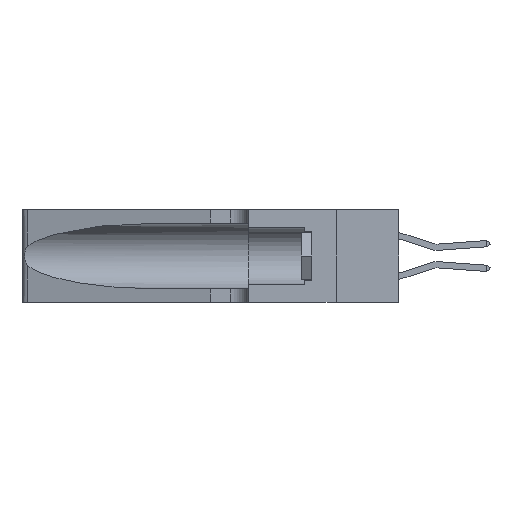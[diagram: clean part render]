
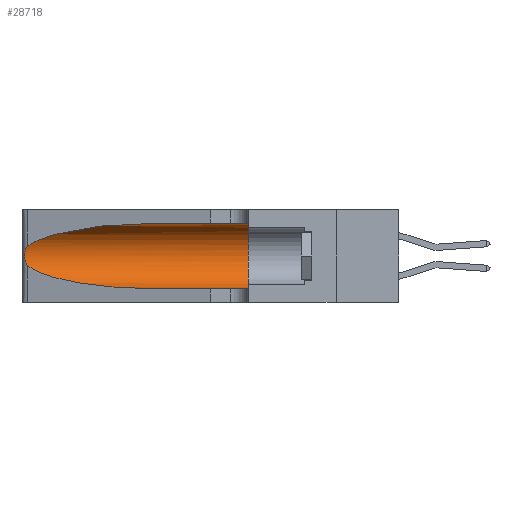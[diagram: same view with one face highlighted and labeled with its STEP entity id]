
A CAD part, left-side view. The second image highlights one B-rep face of the part: STEP entity #28718.
In plain terms, the highlighted cylindrical face has radius 3.308 mm (diameter 6.617 mm), a partial arc.
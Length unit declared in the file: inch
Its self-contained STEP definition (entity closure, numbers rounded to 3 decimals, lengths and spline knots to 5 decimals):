
#351 = VERTEX_POINT ( 'NONE', #17023 ) ;
#1163 = EDGE_CURVE ( 'NONE', #14484, #18772, #7577, .T. ) ;
#1216 = ORIENTED_EDGE ( 'NONE', *, *, #2933, .T. ) ;
#1233 = CARTESIAN_POINT ( 'NONE',  ( 0.1305, 1.61858, 0.05475 ) ) ;
#2181 = CARTESIAN_POINT ( 'NONE',  ( 0.25854, 1.2359, 0.20912 ) ) ;
#2210 = EDGE_LOOP ( 'NONE', ( #8431, #28573, #1216, #13275, #25528, #15955 ) ) ;
#2351 = DIRECTION ( 'NONE',  ( 0., -1., 0. ) ) ;
#2374 = CARTESIAN_POINT ( 'NONE',  ( 0.25487, 1.22718, 0.14631 ) ) ;
#2444 = EDGE_CURVE ( 'NONE', #351, #23136, #7590, .T. ) ;
#2933 = EDGE_CURVE ( 'NONE', #22649, #6682, #25828, .T. ) ;
#4536 = CARTESIAN_POINT ( 'NONE',  ( 0.26075, 1.23896, 0.19203 ) ) ;
#4545 = CARTESIAN_POINT ( 'NONE',  ( 0.2373, 1.15595, 0.28018 ) ) ;
#5528 = CARTESIAN_POINT ( 'NONE',  ( 0.1305, 0.72297, 0.31525 ) ) ;
#6630 = EDGE_CURVE ( 'NONE', #14484, #351, #11268, .T. ) ;
#6682 = VERTEX_POINT ( 'NONE', #26840 ) ;
#6856 = CARTESIAN_POINT ( 'NONE',  ( 0.26017, 1.23833, 0.17102 ) ) ;
#7577 =( BOUNDED_CURVE ( )  B_SPLINE_CURVE ( 3, ( #5528, #20667, #4545, #17344 ),
 .UNSPECIFIED., .F., .F. ) 
 B_SPLINE_CURVE_WITH_KNOTS ( ( 4, 4 ),
 ( 1.5708, 2.84003 ),
 .UNSPECIFIED. ) 
 CURVE ( )  GEOMETRIC_REPRESENTATION_ITEM ( )  RATIONAL_B_SPLINE_CURVE ( ( 1., 0.87, 0.87, 1. ) ) 
 REPRESENTATION_ITEM ( '' )  );
#7590 = CIRCLE ( 'NONE', #27011, 0.13025 ) ;
#8431 = ORIENTED_EDGE ( 'NONE', *, *, #1163, .T. ) ;
#9037 = CARTESIAN_POINT ( 'NONE',  ( 0.25555, 1.22994, 0.2215 ) ) ;
#9132 = CARTESIAN_POINT ( 'NONE',  ( 0.25789, 1.23486, 0.15765 ) ) ;
#10758 = LINE ( 'NONE', #1233, #16496 ) ;
#11268 = LINE ( 'NONE', #13593, #21477 ) ;
#11364 = CARTESIAN_POINT ( 'NONE',  ( 0.25555, 1.22993, 0.14849 ) ) ;
#11855 = AXIS2_PLACEMENT_3D ( 'NONE', #19155, #14835, #17044 ) ;
#13043 = DIRECTION ( 'NONE',  ( 0., 0., 1. ) ) ;
#13275 = ORIENTED_EDGE ( 'NONE', *, *, #23592, .T. ) ;
#13399 = CARTESIAN_POINT ( 'NONE',  ( 0.1305, 0.35, 0.185 ) ) ;
#13593 = CARTESIAN_POINT ( 'NONE',  ( 0.1305, 1.61858, 0.31525 ) ) ;
#13814 = CARTESIAN_POINT ( 'NONE',  ( 0.25487, 1.22718, 0.22369 ) ) ;
#14484 = VERTEX_POINT ( 'NONE', #27884 ) ;
#14698 = DIRECTION ( 'NONE',  ( 0., -1., 0. ) ) ;
#14835 = DIRECTION ( 'NONE',  ( 0., -1., 0. ) ) ;
#15591 = CARTESIAN_POINT ( 'NONE',  ( 0.25787, 1.23484, 0.2124 ) ) ;
#15955 = ORIENTED_EDGE ( 'NONE', *, *, #6630, .F. ) ;
#16496 = VECTOR ( 'NONE', #14698, 39.37008 ) ;
#17023 = CARTESIAN_POINT ( 'NONE',  ( 0.1305, 0.35, 0.31525 ) ) ;
#17044 = DIRECTION ( 'NONE',  ( 0., 0., -1. ) ) ;
#17193 = EDGE_CURVE ( 'NONE', #18772, #22649, #18629, .T. ) ;
#17344 = CARTESIAN_POINT ( 'NONE',  ( 0.25487, 1.22718, 0.22369 ) ) ;
#17785 = CARTESIAN_POINT ( 'NONE',  ( 0.26018, 1.23835, 0.19895 ) ) ;
#18629 = B_SPLINE_CURVE_WITH_KNOTS ( 'NONE', 3,
 ( #24306, #9037, #28663, #15591, #2181, #17785, #4536, #19994, #6856, #22212, #9132, #24398, #11364, #26594 ),
 .UNSPECIFIED., .F., .F.,
 ( 4, 2, 2, 2, 2, 2, 4 ),
 ( 0., 0.00027, 0.00053, 0.00107, 0.0016, 0.00187, 0.00214 ),
 .UNSPECIFIED. ) ;
#18772 = VERTEX_POINT ( 'NONE', #13814 ) ;
#19155 = CARTESIAN_POINT ( 'NONE',  ( 0.1305, 1.61858, 0.185 ) ) ;
#19795 = CARTESIAN_POINT ( 'NONE',  ( 0.1305, 0.35, 0.05475 ) ) ;
#19994 = CARTESIAN_POINT ( 'NONE',  ( 0.26075, 1.23896, 0.178 ) ) ;
#19998 = CYLINDRICAL_SURFACE ( 'NONE', #11855, 0.13025 ) ;
#20667 = CARTESIAN_POINT ( 'NONE',  ( 0.18966, 0.96281, 0.31525 ) ) ;
#21270 = DIRECTION ( 'NONE',  ( 0., 1., 0. ) ) ;
#21477 = VECTOR ( 'NONE', #2351, 39.37008 ) ;
#22212 = CARTESIAN_POINT ( 'NONE',  ( 0.25856, 1.23593, 0.16098 ) ) ;
#22649 = VERTEX_POINT ( 'NONE', #24892 ) ;
#23136 = VERTEX_POINT ( 'NONE', #19795 ) ;
#23592 = EDGE_CURVE ( 'NONE', #6682, #23136, #10758, .T. ) ;
#24053 = CARTESIAN_POINT ( 'NONE',  ( 0.2373, 1.15595, 0.08982 ) ) ;
#24306 = CARTESIAN_POINT ( 'NONE',  ( 0.25487, 1.22718, 0.22369 ) ) ;
#24398 = CARTESIAN_POINT ( 'NONE',  ( 0.25639, 1.23186, 0.15144 ) ) ;
#24892 = CARTESIAN_POINT ( 'NONE',  ( 0.25487, 1.22718, 0.14631 ) ) ;
#25528 = ORIENTED_EDGE ( 'NONE', *, *, #2444, .F. ) ;
#25828 =( BOUNDED_CURVE ( )  B_SPLINE_CURVE ( 3, ( #2374, #24053, #28141, #27008 ),
 .UNSPECIFIED., .F., .F. ) 
 B_SPLINE_CURVE_WITH_KNOTS ( ( 4, 4 ),
 ( 3.44316, 4.71239 ),
 .UNSPECIFIED. ) 
 CURVE ( )  GEOMETRIC_REPRESENTATION_ITEM ( )  RATIONAL_B_SPLINE_CURVE ( ( 1., 0.87, 0.87, 1. ) ) 
 REPRESENTATION_ITEM ( '' )  );
#26502 = FACE_OUTER_BOUND ( 'NONE', #2210, .T. ) ;
#26594 = CARTESIAN_POINT ( 'NONE',  ( 0.25487, 1.22718, 0.14631 ) ) ;
#26840 = CARTESIAN_POINT ( 'NONE',  ( 0.1305, 0.72297, 0.05475 ) ) ;
#27008 = CARTESIAN_POINT ( 'NONE',  ( 0.1305, 0.72297, 0.05475 ) ) ;
#27011 = AXIS2_PLACEMENT_3D ( 'NONE', #13399, #21270, #13043 ) ;
#27884 = CARTESIAN_POINT ( 'NONE',  ( 0.1305, 0.72297, 0.31525 ) ) ;
#28141 = CARTESIAN_POINT ( 'NONE',  ( 0.18966, 0.96281, 0.05475 ) ) ;
#28573 = ORIENTED_EDGE ( 'NONE', *, *, #17193, .T. ) ;
#28663 = CARTESIAN_POINT ( 'NONE',  ( 0.25639, 1.23184, 0.21858 ) ) ;
#28718 = ADVANCED_FACE ( 'NONE', ( #26502 ), #19998, .F. ) ;
